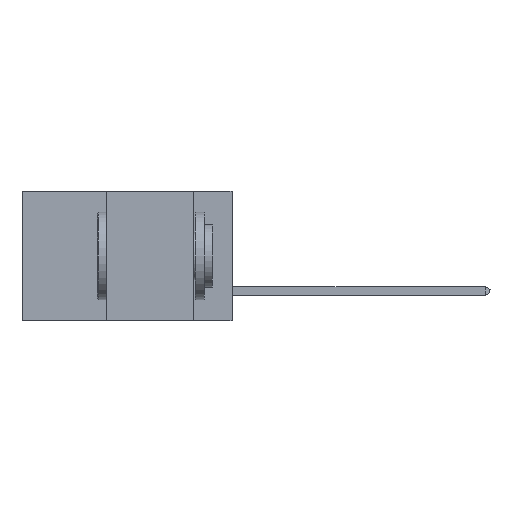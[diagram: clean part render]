
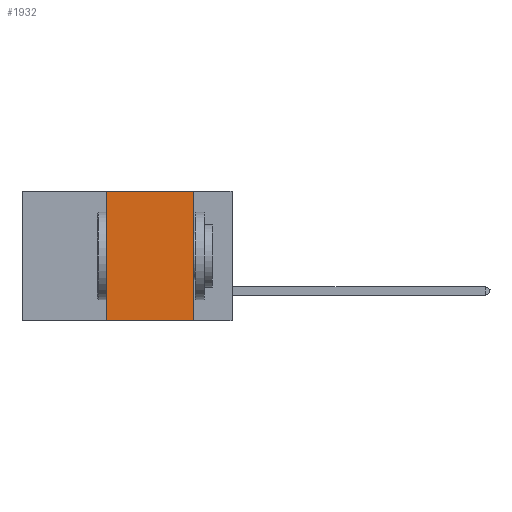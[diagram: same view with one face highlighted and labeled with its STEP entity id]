
A CAD part, left-side view. The second image highlights one B-rep face of the part: STEP entity #1932.
In plain terms, the highlighted planar face has unit normal (-1, 0, 0).
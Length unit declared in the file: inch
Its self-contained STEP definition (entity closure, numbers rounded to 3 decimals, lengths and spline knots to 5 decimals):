
#108 = VECTOR ( 'NONE', #7016, 39.37008 ) ;
#242 = FACE_OUTER_BOUND ( 'NONE', #6452, .T. ) ;
#582 = LINE ( 'NONE', #3471, #9468 ) ;
#626 = AXIS2_PLACEMENT_3D ( 'NONE', #6893, #7802, #3431 ) ;
#786 = PLANE ( 'NONE',  #626 ) ;
#1098 = CARTESIAN_POINT ( 'NONE',  ( 0., 0.11, 0. ) ) ;
#1114 = VERTEX_POINT ( 'NONE', #8063 ) ;
#1426 = VECTOR ( 'NONE', #4958, 39.37008 ) ;
#1671 = VECTOR ( 'NONE', #6315, 39.37008 ) ;
#1932 = ADVANCED_FACE ( 'NONE', ( #242 ), #786, .F. ) ;
#2370 = ORIENTED_EDGE ( 'NONE', *, *, #6474, .F. ) ;
#3103 = EDGE_CURVE ( 'NONE', #6444, #1114, #582, .T. ) ;
#3185 = CARTESIAN_POINT ( 'NONE',  ( 0., 0.6, 0. ) ) ;
#3431 = DIRECTION ( 'NONE',  ( 0., 0., -1. ) ) ;
#3471 = CARTESIAN_POINT ( 'NONE',  ( 0., 0.36, 0. ) ) ;
#3739 = CARTESIAN_POINT ( 'NONE',  ( 0., 0.11, 0. ) ) ;
#4317 = ORIENTED_EDGE ( 'NONE', *, *, #7417, .F. ) ;
#4682 = LINE ( 'NONE', #1098, #108 ) ;
#4733 = CARTESIAN_POINT ( 'NONE',  ( 0., 0.11, -0.37 ) ) ;
#4958 = DIRECTION ( 'NONE',  ( 0., -1., 0. ) ) ;
#6019 = LINE ( 'NONE', #3185, #1426 ) ;
#6315 = DIRECTION ( 'NONE',  ( 0., -1., 0. ) ) ;
#6444 = VERTEX_POINT ( 'NONE', #6689 ) ;
#6452 = EDGE_LOOP ( 'NONE', ( #2370, #4317, #8617, #10306 ) ) ;
#6474 = EDGE_CURVE ( 'NONE', #8275, #7295, #4682, .T. ) ;
#6689 = CARTESIAN_POINT ( 'NONE',  ( 0., 0.36, -0.37 ) ) ;
#6893 = CARTESIAN_POINT ( 'NONE',  ( 0., 0.6, 0. ) ) ;
#7016 = DIRECTION ( 'NONE',  ( 0., 0., -1. ) ) ;
#7271 = CARTESIAN_POINT ( 'NONE',  ( 0., 0.6, -0.37 ) ) ;
#7295 = VERTEX_POINT ( 'NONE', #4733 ) ;
#7417 = EDGE_CURVE ( 'NONE', #1114, #8275, #6019, .T. ) ;
#7802 = DIRECTION ( 'NONE',  ( 1., 0., 0. ) ) ;
#8063 = CARTESIAN_POINT ( 'NONE',  ( 0., 0.36, 0. ) ) ;
#8275 = VERTEX_POINT ( 'NONE', #3739 ) ;
#8617 = ORIENTED_EDGE ( 'NONE', *, *, #3103, .F. ) ;
#9120 = EDGE_CURVE ( 'NONE', #6444, #7295, #10881, .T. ) ;
#9468 = VECTOR ( 'NONE', #9561, 39.37008 ) ;
#9561 = DIRECTION ( 'NONE',  ( 0., 0., 1. ) ) ;
#10306 = ORIENTED_EDGE ( 'NONE', *, *, #9120, .T. ) ;
#10881 = LINE ( 'NONE', #7271, #1671 ) ;
